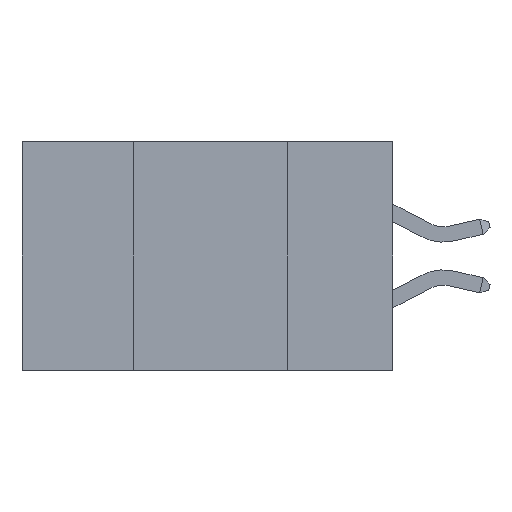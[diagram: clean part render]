
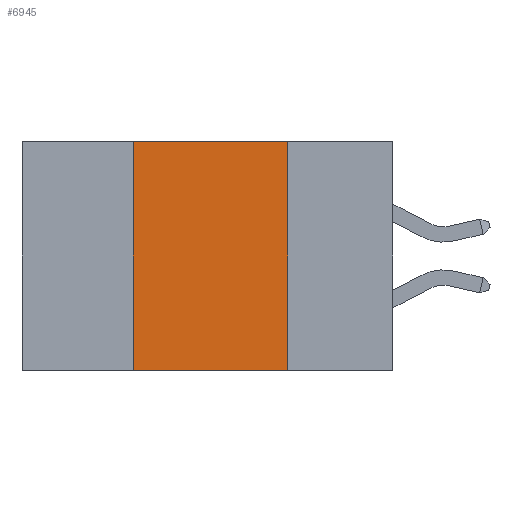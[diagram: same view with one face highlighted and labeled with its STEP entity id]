
A CAD part, left-side view. The second image highlights one B-rep face of the part: STEP entity #6945.
In plain terms, the highlighted planar face has unit normal (-1, 0, 0).
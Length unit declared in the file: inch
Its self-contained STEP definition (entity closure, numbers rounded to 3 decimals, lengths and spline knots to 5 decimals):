
#186 = DIRECTION ( 'NONE',  ( 0., 0., 1. ) ) ;
#643 = CARTESIAN_POINT ( 'NONE',  ( 0., 0.6, 0. ) ) ;
#968 = CARTESIAN_POINT ( 'NONE',  ( 0., 0.6, 0. ) ) ;
#1134 = DIRECTION ( 'NONE',  ( 0., 0., -1. ) ) ;
#1181 = CARTESIAN_POINT ( 'NONE',  ( 0., 0.17, 0. ) ) ;
#1688 = VECTOR ( 'NONE', #1134, 39.37008 ) ;
#1820 = DIRECTION ( 'NONE',  ( 1., 0., 0. ) ) ;
#2013 = EDGE_CURVE ( 'NONE', #3543, #6123, #10770, .T. ) ;
#2204 = VERTEX_POINT ( 'NONE', #9379 ) ;
#2528 = ORIENTED_EDGE ( 'NONE', *, *, #11063, .F. ) ;
#2827 = CARTESIAN_POINT ( 'NONE',  ( 0., 0.42, 0. ) ) ;
#3254 = DIRECTION ( 'NONE',  ( 0., -1., 0. ) ) ;
#3543 = VERTEX_POINT ( 'NONE', #9213 ) ;
#3593 = EDGE_CURVE ( 'NONE', #2204, #3543, #9030, .T. ) ;
#4086 = LINE ( 'NONE', #2827, #6941 ) ;
#4208 = VECTOR ( 'NONE', #10268, 39.37008 ) ;
#4285 = ORIENTED_EDGE ( 'NONE', *, *, #2013, .F. ) ;
#4326 = EDGE_CURVE ( 'NONE', #6631, #6123, #10726, .T. ) ;
#4819 = ORIENTED_EDGE ( 'NONE', *, *, #4326, .T. ) ;
#4956 = FACE_OUTER_BOUND ( 'NONE', #5386, .T. ) ;
#5386 = EDGE_LOOP ( 'NONE', ( #4285, #11052, #2528, #4819 ) ) ;
#6116 = PLANE ( 'NONE',  #9161 ) ;
#6123 = VERTEX_POINT ( 'NONE', #6681 ) ;
#6597 = CARTESIAN_POINT ( 'NONE',  ( 0., 0.42, -0.37 ) ) ;
#6631 = VERTEX_POINT ( 'NONE', #6597 ) ;
#6681 = CARTESIAN_POINT ( 'NONE',  ( 0., 0.17, -0.37 ) ) ;
#6941 = VECTOR ( 'NONE', #186, 39.37008 ) ;
#6945 = ADVANCED_FACE ( 'NONE', ( #4956 ), #6116, .F. ) ;
#7820 = CARTESIAN_POINT ( 'NONE',  ( 0., 0.6, -0.37 ) ) ;
#7926 = DIRECTION ( 'NONE',  ( 0., 0., -1. ) ) ;
#8956 = VECTOR ( 'NONE', #3254, 39.37008 ) ;
#9030 = LINE ( 'NONE', #643, #8956 ) ;
#9161 = AXIS2_PLACEMENT_3D ( 'NONE', #968, #1820, #7926 ) ;
#9213 = CARTESIAN_POINT ( 'NONE',  ( 0., 0.17, 0. ) ) ;
#9379 = CARTESIAN_POINT ( 'NONE',  ( 0., 0.42, 0. ) ) ;
#10268 = DIRECTION ( 'NONE',  ( 0., -1., 0. ) ) ;
#10726 = LINE ( 'NONE', #7820, #4208 ) ;
#10770 = LINE ( 'NONE', #1181, #1688 ) ;
#11052 = ORIENTED_EDGE ( 'NONE', *, *, #3593, .F. ) ;
#11063 = EDGE_CURVE ( 'NONE', #6631, #2204, #4086, .T. ) ;
